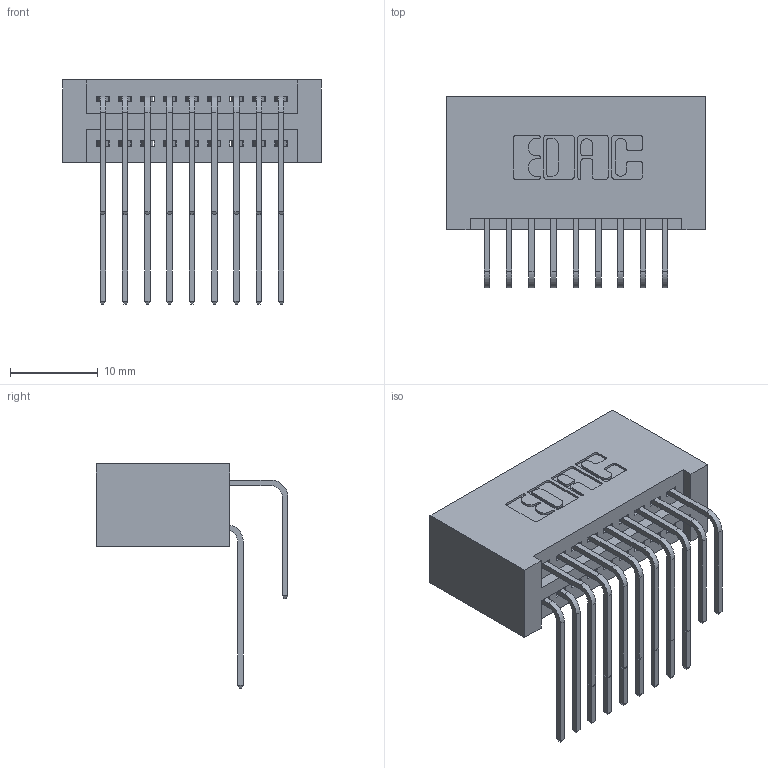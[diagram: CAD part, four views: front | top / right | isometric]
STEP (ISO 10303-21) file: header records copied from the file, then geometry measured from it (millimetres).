
FILE_DESCRIPTION (( 'STEP AP203' ), '1' );
FILE_NAME ('395-018-558-201.STEP', '2018-11-07T03:43:48', ( '' ), ( '' ), 'SwSTEP 2.0', 'SolidWorks 2016', '' );
FILE_SCHEMA (( 'CONFIG_CONTROL_DESIGN' ));
Length unit declared in the file: inch
Products named in the file (4): 395-018-558-201; 345 Part_No Mounting Lugs; 345-292-001_558 Tail - 2; 345-292-001_558 559 Tail - 1
Assembly tree (19 placements, depth 2):
  395-018-558-201
    345 Part_No Mounting Lugs
    345-292-001_558 559 Tail - 1  x9
    345-292-001_558 Tail - 2  x9
Bounding box: 29.46 x 21.83 x 25.53 mm (x, y, z)
Volume: 3275.6 mm3; surface area: 4994.3 mm2
Topology: 19 solids, 19 shells, 1054 faces, 3107 edges, 2046 vertices
Faces by surface type: plane 706, cylinder 348
Entity records: 12879 total; most frequent: CARTESIAN_POINT 2235, ORIENTED_EDGE 2118, DIRECTION 1979, EDGE_CURVE 1059, VECTOR 859, LINE 859, VERTEX_POINT 702, AXIS2_PLACEMENT_3D 560
